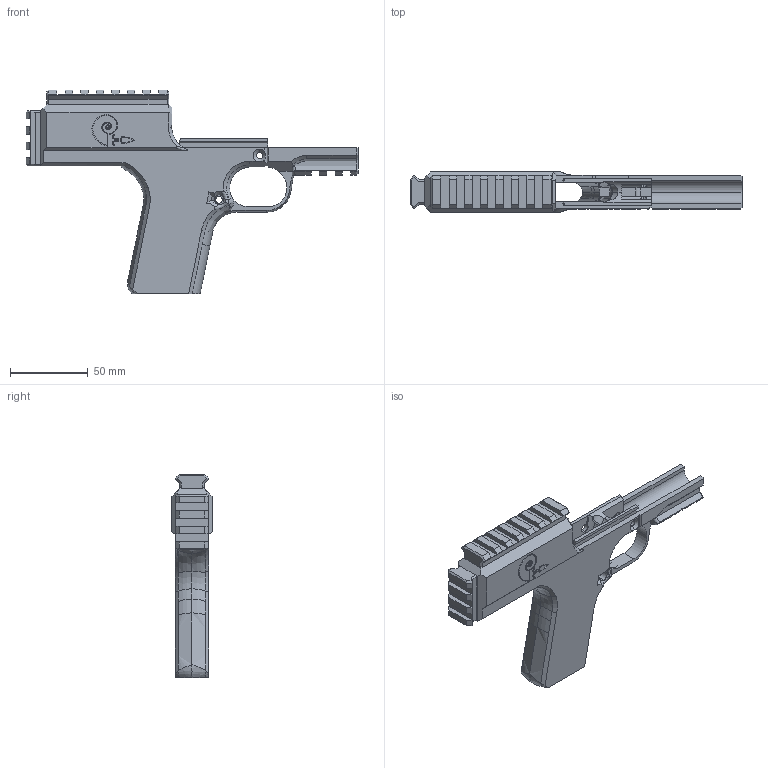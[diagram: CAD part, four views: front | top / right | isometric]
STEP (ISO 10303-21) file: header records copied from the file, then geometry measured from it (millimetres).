
FILE_DESCRIPTION (( 'STEP AP203' ), '1' );
FILE_NAME ('Nautilus-TT v1.0.STEP', '2020-10-26T16:59:21', ( '' ), ( '' ), 'SwSTEP 2.0', 'SolidWorks 2019', '' );
FILE_SCHEMA (( 'CONFIG_CONTROL_DESIGN' ));
Length unit declared in the file: millimetre
Products named in the file (1): Nautilus-TT v1.0
Bounding box: 213.4 x 25.8 x 130.8 mm (x, y, z)
Volume: 119105.5 mm3; surface area: 59069.2 mm2
Topology: 1 solids, 1 shells, 603 faces, 1686 edges, 1082 vertices
Faces by surface type: plane 390, bspline 95, cylinder 88, cone 26, torus 4
Entity records: 25405 total; most frequent: CARTESIAN_POINT 10680, ORIENTED_EDGE 3372, DIRECTION 2610, EDGE_CURVE 1686, LINE 1132, VECTOR 1132, VERTEX_POINT 1082, AXIS2_PLACEMENT_3D 739
